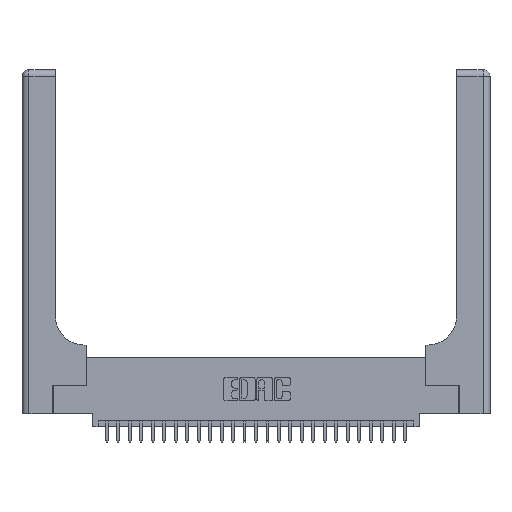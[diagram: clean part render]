
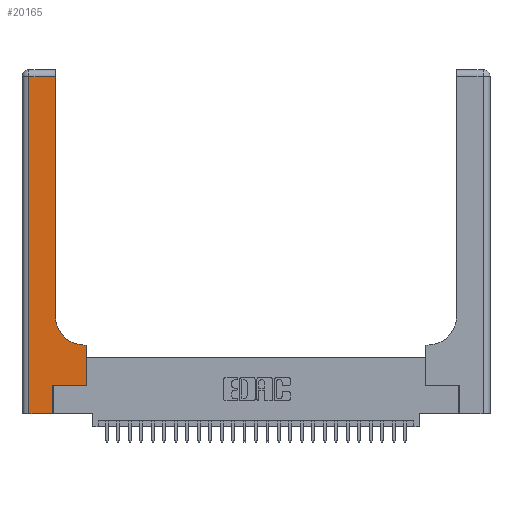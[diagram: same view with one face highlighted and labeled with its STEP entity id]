
A CAD part, top view. The second image highlights one B-rep face of the part: STEP entity #20165.
In plain terms, the highlighted planar face has unit normal (0, 0, 1).
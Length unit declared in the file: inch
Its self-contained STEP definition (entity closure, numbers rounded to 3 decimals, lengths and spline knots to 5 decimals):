
#273 = CARTESIAN_POINT ( 'NONE',  ( 0.269, 0.25, 0.37 ) ) ;
#320 = LINE ( 'NONE', #13697, #23035 ) ;
#512 = CARTESIAN_POINT ( 'NONE',  ( 0.2915, 0.6, 0.37 ) ) ;
#556 = ORIENTED_EDGE ( 'NONE', *, *, #22136, .T. ) ;
#997 = CARTESIAN_POINT ( 'NONE',  ( 0.5585, 0.6, 0.37 ) ) ;
#2744 = DIRECTION ( 'NONE',  ( -1., 0., 0. ) ) ;
#2811 = VERTEX_POINT ( 'NONE', #5374 ) ;
#3868 = CARTESIAN_POINT ( 'NONE',  ( 0.5415, 0.6, 0.37 ) ) ;
#4170 = ORIENTED_EDGE ( 'NONE', *, *, #5734, .T. ) ;
#4279 = CARTESIAN_POINT ( 'NONE',  ( 0., 2.94, 0.37 ) ) ;
#4399 = VECTOR ( 'NONE', #12932, 39.37008 ) ;
#4775 = PLANE ( 'NONE',  #20539 ) ;
#5374 = CARTESIAN_POINT ( 'NONE',  ( 0.269, 0., 0.37 ) ) ;
#5670 = CARTESIAN_POINT ( 'NONE',  ( 0., 0., 0.37 ) ) ;
#5734 = EDGE_CURVE ( 'NONE', #6211, #21963, #320, .T. ) ;
#6211 = VERTEX_POINT ( 'NONE', #273 ) ;
#6486 = DIRECTION ( 'NONE',  ( -1., 0., 0. ) ) ;
#7048 = DIRECTION ( 'NONE',  ( 0., 0., -1. ) ) ;
#7772 = CARTESIAN_POINT ( 'NONE',  ( 0.06, 2.94, 0.37 ) ) ;
#8087 = VECTOR ( 'NONE', #20987, 39.37008 ) ;
#8590 = VECTOR ( 'NONE', #21914, 39.37008 ) ;
#9079 = VERTEX_POINT ( 'NONE', #10918 ) ;
#9740 = AXIS2_PLACEMENT_3D ( 'NONE', #23511, #10332, #25724 ) ;
#9825 = LINE ( 'NONE', #4279, #26728 ) ;
#9887 = CARTESIAN_POINT ( 'NONE',  ( 0.2915, 2.94, 0.37 ) ) ;
#9969 = VECTOR ( 'NONE', #2744, 39.37008 ) ;
#10332 = DIRECTION ( 'NONE',  ( 0., 0., -1. ) ) ;
#10872 = DIRECTION ( 'NONE',  ( 0., 1., 0. ) ) ;
#10918 = CARTESIAN_POINT ( 'NONE',  ( 0.06, 0., 0.37 ) ) ;
#12230 = VECTOR ( 'NONE', #15097, 39.37008 ) ;
#12892 = CARTESIAN_POINT ( 'NONE',  ( 0.2915, 3., 0.37 ) ) ;
#12932 = DIRECTION ( 'NONE',  ( 0., -1., 0. ) ) ;
#13109 = ORIENTED_EDGE ( 'NONE', *, *, #13556, .T. ) ;
#13556 = EDGE_CURVE ( 'NONE', #19101, #9079, #27803, .T. ) ;
#13697 = CARTESIAN_POINT ( 'NONE',  ( 0.269, 0.25, 0.37 ) ) ;
#14103 = CIRCLE ( 'NONE', #9740, 0.25 ) ;
#14560 = EDGE_CURVE ( 'NONE', #9079, #2811, #24959, .T. ) ;
#15097 = DIRECTION ( 'NONE',  ( 0., 1., 0. ) ) ;
#15373 = CARTESIAN_POINT ( 'NONE',  ( 0.5585, 0.25, 0.37 ) ) ;
#15508 = ORIENTED_EDGE ( 'NONE', *, *, #17619, .T. ) ;
#15647 = CARTESIAN_POINT ( 'NONE',  ( 0.2915, 0.85, 0.37 ) ) ;
#16210 = EDGE_LOOP ( 'NONE', ( #15508, #22698, #13109, #18905, #25487, #4170, #22050, #556, #18167 ) ) ;
#16453 = VERTEX_POINT ( 'NONE', #15647 ) ;
#17026 = EDGE_CURVE ( 'NONE', #21091, #19101, #9825, .T. ) ;
#17241 = CARTESIAN_POINT ( 'NONE',  ( 0.06, 3., 0.37 ) ) ;
#17372 = LINE ( 'NONE', #21809, #27733 ) ;
#17619 = EDGE_CURVE ( 'NONE', #16453, #21091, #23215, .T. ) ;
#17659 = EDGE_CURVE ( 'NONE', #2811, #6211, #17372, .T. ) ;
#18167 = ORIENTED_EDGE ( 'NONE', *, *, #22436, .T. ) ;
#18905 = ORIENTED_EDGE ( 'NONE', *, *, #14560, .T. ) ;
#19101 = VERTEX_POINT ( 'NONE', #7772 ) ;
#19692 = CARTESIAN_POINT ( 'NONE',  ( 0.5585, 0.25, 0.37 ) ) ;
#20165 = ADVANCED_FACE ( 'NONE', ( #25206 ), #4775, .F. ) ;
#20193 = CARTESIAN_POINT ( 'NONE',  ( 0., 3., 0.37 ) ) ;
#20539 = AXIS2_PLACEMENT_3D ( 'NONE', #20193, #7048, #22433 ) ;
#20987 = DIRECTION ( 'NONE',  ( 1., 0., 0. ) ) ;
#21091 = VERTEX_POINT ( 'NONE', #9887 ) ;
#21809 = CARTESIAN_POINT ( 'NONE',  ( 0.269, 0., 0.37 ) ) ;
#21914 = DIRECTION ( 'NONE',  ( 0., 1., 0. ) ) ;
#21963 = VERTEX_POINT ( 'NONE', #15373 ) ;
#22050 = ORIENTED_EDGE ( 'NONE', *, *, #23353, .T. ) ;
#22136 = EDGE_CURVE ( 'NONE', #23690, #23212, #27558, .T. ) ;
#22433 = DIRECTION ( 'NONE',  ( -1., 0., 0. ) ) ;
#22436 = EDGE_CURVE ( 'NONE', #23212, #16453, #14103, .T. ) ;
#22698 = ORIENTED_EDGE ( 'NONE', *, *, #17026, .T. ) ;
#23035 = VECTOR ( 'NONE', #26973, 39.37008 ) ;
#23212 = VERTEX_POINT ( 'NONE', #3868 ) ;
#23215 = LINE ( 'NONE', #12892, #12230 ) ;
#23353 = EDGE_CURVE ( 'NONE', #21963, #23690, #26153, .T. ) ;
#23511 = CARTESIAN_POINT ( 'NONE',  ( 0.5415, 0.85, 0.37 ) ) ;
#23690 = VERTEX_POINT ( 'NONE', #997 ) ;
#24959 = LINE ( 'NONE', #5670, #8087 ) ;
#25206 = FACE_OUTER_BOUND ( 'NONE', #16210, .T. ) ;
#25487 = ORIENTED_EDGE ( 'NONE', *, *, #17659, .T. ) ;
#25724 = DIRECTION ( 'NONE',  ( 1., 0., 0. ) ) ;
#26153 = LINE ( 'NONE', #19692, #8590 ) ;
#26728 = VECTOR ( 'NONE', #6486, 39.37008 ) ;
#26973 = DIRECTION ( 'NONE',  ( 1., 0., 0. ) ) ;
#27558 = LINE ( 'NONE', #512, #9969 ) ;
#27733 = VECTOR ( 'NONE', #10872, 39.37008 ) ;
#27803 = LINE ( 'NONE', #17241, #4399 ) ;
